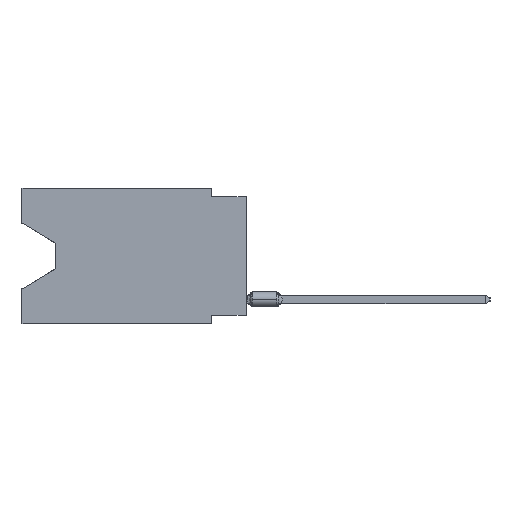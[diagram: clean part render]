
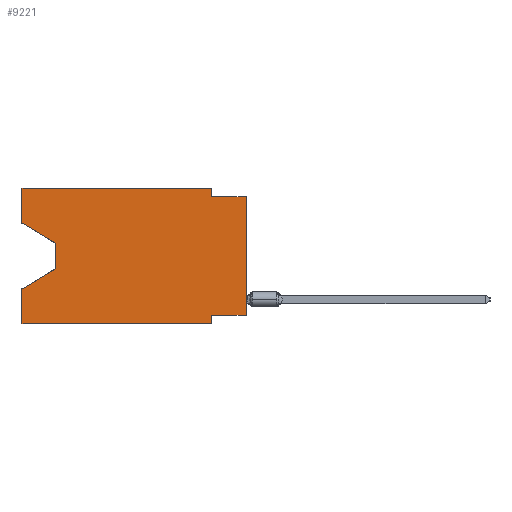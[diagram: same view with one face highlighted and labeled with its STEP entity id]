
A CAD part, left-side view. The second image highlights one B-rep face of the part: STEP entity #9221.
In plain terms, the highlighted planar face has unit normal (-1, 0, 0).
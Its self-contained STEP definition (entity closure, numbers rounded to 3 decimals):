
#197 = VECTOR ( 'NONE', #16756, 1000. ) ;
#544 = FACE_OUTER_BOUND ( 'NONE', #10341, .T. ) ;
#1368 = CARTESIAN_POINT ( 'NONE',  ( 0., 0., -9.271 ) ) ;
#1524 = CARTESIAN_POINT ( 'NONE',  ( 0., 16.383, 0. ) ) ;
#2001 = VECTOR ( 'NONE', #10741, 1000. ) ;
#2342 = DIRECTION ( 'NONE',  ( 0., 0., 1. ) ) ;
#2439 = ORIENTED_EDGE ( 'NONE', *, *, #25308, .T. ) ;
#3122 = VERTEX_POINT ( 'NONE', #17479 ) ;
#3691 = VECTOR ( 'NONE', #41462, 1000. ) ;
#3950 = CARTESIAN_POINT ( 'NONE',  ( 0., 13.97, -5.893 ) ) ;
#4607 = EDGE_CURVE ( 'NONE', #34318, #46459, #31952, .T. ) ;
#4649 = DIRECTION ( 'NONE',  ( 0., 0., -1. ) ) ;
#6473 = CARTESIAN_POINT ( 'NONE',  ( 0., 13.97, -4.013 ) ) ;
#6685 = EDGE_CURVE ( 'NONE', #16933, #14643, #10174, .T. ) ;
#6939 = CARTESIAN_POINT ( 'NONE',  ( 0., 2.54, 0. ) ) ;
#7394 = VECTOR ( 'NONE', #32788, 1000. ) ;
#7695 = CARTESIAN_POINT ( 'NONE',  ( 0., 16.383, -9.906 ) ) ;
#9221 = ADVANCED_FACE ( 'NONE', ( #544 ), #16641, .F. ) ;
#10048 = ORIENTED_EDGE ( 'NONE', *, *, #20152, .T. ) ;
#10174 = LINE ( 'NONE', #40424, #21355 ) ;
#10341 = EDGE_LOOP ( 'NONE', ( #10828, #22514, #2439, #16975, #42258, #10734, #16725, #10048, #48121, #28497, #22181, #24756 ) ) ;
#10734 = ORIENTED_EDGE ( 'NONE', *, *, #6685, .F. ) ;
#10741 = DIRECTION ( 'NONE',  ( 0., 0., -1. ) ) ;
#10828 = ORIENTED_EDGE ( 'NONE', *, *, #24490, .T. ) ;
#11024 = VECTOR ( 'NONE', #47028, 1000. ) ;
#11492 = EDGE_CURVE ( 'NONE', #40822, #25520, #46702, .T. ) ;
#12057 = EDGE_CURVE ( 'NONE', #25520, #38945, #13702, .T. ) ;
#12389 = EDGE_CURVE ( 'NONE', #3122, #16933, #13404, .T. ) ;
#12493 = LINE ( 'NONE', #32384, #11024 ) ;
#12588 = DIRECTION ( 'NONE',  ( 0., 0., -1. ) ) ;
#12832 = CARTESIAN_POINT ( 'NONE',  ( 0., 16.383, 0. ) ) ;
#13404 = LINE ( 'NONE', #1368, #7394 ) ;
#13702 = LINE ( 'NONE', #40669, #197 ) ;
#13910 = VECTOR ( 'NONE', #43572, 1000. ) ;
#14643 = VERTEX_POINT ( 'NONE', #15278 ) ;
#14919 = VECTOR ( 'NONE', #46328, 1000. ) ;
#15268 = DIRECTION ( 'NONE',  ( 0., -0.855, -0.519 ) ) ;
#15278 = CARTESIAN_POINT ( 'NONE',  ( 0., 2.54, -9.906 ) ) ;
#15703 = VERTEX_POINT ( 'NONE', #45497 ) ;
#15970 = CARTESIAN_POINT ( 'NONE',  ( 0., 2.54, 0. ) ) ;
#16101 = AXIS2_PLACEMENT_3D ( 'NONE', #12832, #16883, #12588 ) ;
#16234 = EDGE_CURVE ( 'NONE', #34318, #14643, #46240, .T. ) ;
#16641 = PLANE ( 'NONE',  #16101 ) ;
#16725 = ORIENTED_EDGE ( 'NONE', *, *, #12389, .F. ) ;
#16756 = DIRECTION ( 'NONE',  ( 0., -1., 0. ) ) ;
#16883 = DIRECTION ( 'NONE',  ( 1., 0., 0. ) ) ;
#16933 = VERTEX_POINT ( 'NONE', #37072 ) ;
#16975 = ORIENTED_EDGE ( 'NONE', *, *, #4607, .F. ) ;
#17479 = CARTESIAN_POINT ( 'NONE',  ( 0., 0., -9.271 ) ) ;
#18151 = CARTESIAN_POINT ( 'NONE',  ( 0., 13.97, -4.013 ) ) ;
#18338 = CARTESIAN_POINT ( 'NONE',  ( 0., 0., -0.635 ) ) ;
#20152 = EDGE_CURVE ( 'NONE', #3122, #38945, #24990, .T. ) ;
#20868 = CARTESIAN_POINT ( 'NONE',  ( 0., 2.54, -0.635 ) ) ;
#21342 = LINE ( 'NONE', #6473, #2001 ) ;
#21355 = VECTOR ( 'NONE', #43958, 1000. ) ;
#22181 = ORIENTED_EDGE ( 'NONE', *, *, #28036, .F. ) ;
#22255 = VECTOR ( 'NONE', #29688, 1000. ) ;
#22514 = ORIENTED_EDGE ( 'NONE', *, *, #45013, .T. ) ;
#23589 = VERTEX_POINT ( 'NONE', #27877 ) ;
#24490 = EDGE_CURVE ( 'NONE', #15703, #30787, #38691, .T. ) ;
#24756 = ORIENTED_EDGE ( 'NONE', *, *, #27111, .F. ) ;
#24990 = LINE ( 'NONE', #36815, #49151 ) ;
#25308 = EDGE_CURVE ( 'NONE', #28616, #46459, #45822, .T. ) ;
#25520 = VERTEX_POINT ( 'NONE', #20868 ) ;
#27111 = EDGE_CURVE ( 'NONE', #15703, #23589, #12493, .T. ) ;
#27877 = CARTESIAN_POINT ( 'NONE',  ( 0., 16.383, 0. ) ) ;
#28036 = EDGE_CURVE ( 'NONE', #23589, #40822, #37500, .T. ) ;
#28497 = ORIENTED_EDGE ( 'NONE', *, *, #11492, .F. ) ;
#28616 = VERTEX_POINT ( 'NONE', #3950 ) ;
#29688 = DIRECTION ( 'NONE',  ( 0., -1., 0. ) ) ;
#30787 = VERTEX_POINT ( 'NONE', #18151 ) ;
#31603 = VECTOR ( 'NONE', #15268, 1000. ) ;
#31952 = LINE ( 'NONE', #1524, #13910 ) ;
#32384 = CARTESIAN_POINT ( 'NONE',  ( 0., 16.383, 0. ) ) ;
#32788 = DIRECTION ( 'NONE',  ( 0., 1., 0. ) ) ;
#34318 = VERTEX_POINT ( 'NONE', #38978 ) ;
#36150 = CARTESIAN_POINT ( 'NONE',  ( 0., 16.383, -7.36 ) ) ;
#36343 = VECTOR ( 'NONE', #4649, 1000. ) ;
#36815 = CARTESIAN_POINT ( 'NONE',  ( 0., 0., 0. ) ) ;
#37072 = CARTESIAN_POINT ( 'NONE',  ( 0., 2.54, -9.271 ) ) ;
#37500 = LINE ( 'NONE', #48605, #22255 ) ;
#38269 = CARTESIAN_POINT ( 'NONE',  ( 0., 13.97, -5.893 ) ) ;
#38691 = LINE ( 'NONE', #45508, #31603 ) ;
#38945 = VERTEX_POINT ( 'NONE', #18338 ) ;
#38978 = CARTESIAN_POINT ( 'NONE',  ( 0., 16.383, -9.906 ) ) ;
#40424 = CARTESIAN_POINT ( 'NONE',  ( 0., 2.54, -9.906 ) ) ;
#40669 = CARTESIAN_POINT ( 'NONE',  ( 0., 0., -0.635 ) ) ;
#40822 = VERTEX_POINT ( 'NONE', #6939 ) ;
#41462 = DIRECTION ( 'NONE',  ( 0., -1., 0. ) ) ;
#42258 = ORIENTED_EDGE ( 'NONE', *, *, #16234, .T. ) ;
#43572 = DIRECTION ( 'NONE',  ( 0., 0., 1. ) ) ;
#43958 = DIRECTION ( 'NONE',  ( 0., 0., -1. ) ) ;
#45013 = EDGE_CURVE ( 'NONE', #30787, #28616, #21342, .T. ) ;
#45497 = CARTESIAN_POINT ( 'NONE',  ( 0., 16.383, -2.546 ) ) ;
#45508 = CARTESIAN_POINT ( 'NONE',  ( 0., 16.383, -2.546 ) ) ;
#45822 = LINE ( 'NONE', #38269, #14919 ) ;
#46240 = LINE ( 'NONE', #7695, #3691 ) ;
#46328 = DIRECTION ( 'NONE',  ( 0., 0.855, -0.519 ) ) ;
#46459 = VERTEX_POINT ( 'NONE', #36150 ) ;
#46702 = LINE ( 'NONE', #15970, #36343 ) ;
#47028 = DIRECTION ( 'NONE',  ( 0., 0., 1. ) ) ;
#48121 = ORIENTED_EDGE ( 'NONE', *, *, #12057, .F. ) ;
#48605 = CARTESIAN_POINT ( 'NONE',  ( 0., 16.383, 0. ) ) ;
#49151 = VECTOR ( 'NONE', #2342, 1000. ) ;
